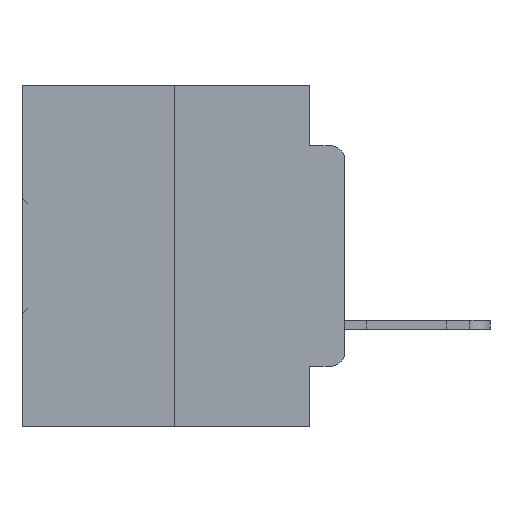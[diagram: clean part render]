
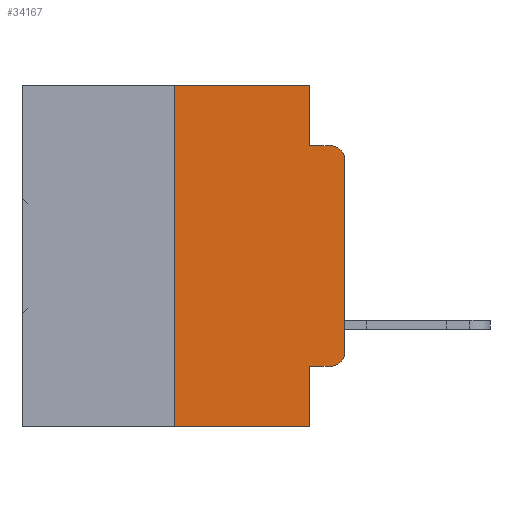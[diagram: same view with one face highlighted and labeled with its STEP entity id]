
A CAD part, left-side view. The second image highlights one B-rep face of the part: STEP entity #34167.
In plain terms, the highlighted planar face has unit normal (-1, 0, 0).
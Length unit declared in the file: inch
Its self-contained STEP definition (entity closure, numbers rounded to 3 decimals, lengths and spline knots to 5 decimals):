
#815 = VERTEX_POINT ( 'NONE', #9999 ) ;
#1784 = AXIS2_PLACEMENT_3D ( 'NONE', #13565, #32236, #16232 ) ;
#1846 = LINE ( 'NONE', #5525, #16604 ) ;
#2454 = CARTESIAN_POINT ( 'NONE',  ( 0., 0.473, -0.5 ) ) ;
#2669 = CARTESIAN_POINT ( 'NONE',  ( 0., 0.051, 0. ) ) ;
#2680 = VERTEX_POINT ( 'NONE', #14502 ) ;
#3505 = ORIENTED_EDGE ( 'NONE', *, *, #15313, .F. ) ;
#3794 = DIRECTION ( 'NONE',  ( 0., -1., 0. ) ) ;
#3886 = EDGE_CURVE ( 'NONE', #815, #17534, #33756, .T. ) ;
#4119 = CIRCLE ( 'NONE', #1784, 0.02 ) ;
#4231 = ORIENTED_EDGE ( 'NONE', *, *, #27863, .F. ) ;
#4337 = CARTESIAN_POINT ( 'NONE',  ( 0., 0.25, 0. ) ) ;
#5525 = CARTESIAN_POINT ( 'NONE',  ( 0., 0., 0. ) ) ;
#6463 = CARTESIAN_POINT ( 'NONE',  ( 0., 0.051, 0. ) ) ;
#6866 = VERTEX_POINT ( 'NONE', #31218 ) ;
#7298 = FACE_OUTER_BOUND ( 'NONE', #7932, .T. ) ;
#7543 = CARTESIAN_POINT ( 'NONE',  ( 0., 0., -0.1085 ) ) ;
#7589 = CARTESIAN_POINT ( 'NONE',  ( 0., 0., -0.3915 ) ) ;
#7918 = EDGE_CURVE ( 'NONE', #25588, #6866, #33479, .T. ) ;
#7932 = EDGE_LOOP ( 'NONE', ( #9572, #29184, #14953, #4231, #29340, #10903, #31826, #3505, #14131, #22045 ) ) ;
#8846 = CARTESIAN_POINT ( 'NONE',  ( 0., 0.051, -0.0885 ) ) ;
#9166 = DIRECTION ( 'NONE',  ( -1., 0., 0. ) ) ;
#9572 = ORIENTED_EDGE ( 'NONE', *, *, #12365, .T. ) ;
#9704 = AXIS2_PLACEMENT_3D ( 'NONE', #34174, #26301, #10127 ) ;
#9999 = CARTESIAN_POINT ( 'NONE',  ( 0., 0.051, -0.0885 ) ) ;
#10127 = DIRECTION ( 'NONE',  ( 0., 0., -1. ) ) ;
#10320 = DIRECTION ( 'NONE',  ( 0., -1., 0. ) ) ;
#10903 = ORIENTED_EDGE ( 'NONE', *, *, #7918, .F. ) ;
#10965 = EDGE_CURVE ( 'NONE', #11527, #17534, #4119, .T. ) ;
#11016 = VERTEX_POINT ( 'NONE', #32355 ) ;
#11527 = VERTEX_POINT ( 'NONE', #7543 ) ;
#12365 = EDGE_CURVE ( 'NONE', #23808, #11527, #1846, .T. ) ;
#12537 = LINE ( 'NONE', #17525, #17151 ) ;
#12842 = CARTESIAN_POINT ( 'NONE',  ( 0., 0.051, 0. ) ) ;
#13093 = EDGE_CURVE ( 'NONE', #25588, #21422, #21567, .T. ) ;
#13341 = VECTOR ( 'NONE', #33465, 39.37008 ) ;
#13565 = CARTESIAN_POINT ( 'NONE',  ( 0., 0.02, -0.1085 ) ) ;
#14131 = ORIENTED_EDGE ( 'NONE', *, *, #34041, .T. ) ;
#14473 = VECTOR ( 'NONE', #21647, 39.37008 ) ;
#14502 = CARTESIAN_POINT ( 'NONE',  ( 0., 0.051, -0.4115 ) ) ;
#14953 = ORIENTED_EDGE ( 'NONE', *, *, #3886, .F. ) ;
#15313 = EDGE_CURVE ( 'NONE', #2680, #21422, #33087, .T. ) ;
#15540 = DIRECTION ( 'NONE',  ( 0., 0., -1. ) ) ;
#16038 = CARTESIAN_POINT ( 'NONE',  ( 0., 0.051, -0.5 ) ) ;
#16232 = DIRECTION ( 'NONE',  ( 0., 0., -1. ) ) ;
#16604 = VECTOR ( 'NONE', #24638, 39.37008 ) ;
#16942 = VECTOR ( 'NONE', #23883, 39.37008 ) ;
#17151 = VECTOR ( 'NONE', #3794, 39.37008 ) ;
#17525 = CARTESIAN_POINT ( 'NONE',  ( 0., 0.051, -0.4115 ) ) ;
#17534 = VERTEX_POINT ( 'NONE', #20799 ) ;
#18224 = PLANE ( 'NONE',  #9704 ) ;
#18900 = VECTOR ( 'NONE', #15540, 39.37008 ) ;
#19289 = VECTOR ( 'NONE', #23483, 39.37008 ) ;
#19571 = VECTOR ( 'NONE', #10320, 39.37008 ) ;
#20799 = CARTESIAN_POINT ( 'NONE',  ( 0., 0.02, -0.0885 ) ) ;
#21422 = VERTEX_POINT ( 'NONE', #16038 ) ;
#21567 = LINE ( 'NONE', #2454, #14473 ) ;
#21647 = DIRECTION ( 'NONE',  ( 0., -1., 0. ) ) ;
#22045 = ORIENTED_EDGE ( 'NONE', *, *, #27207, .T. ) ;
#23483 = DIRECTION ( 'NONE',  ( 0., 0., 1. ) ) ;
#23808 = VERTEX_POINT ( 'NONE', #7589 ) ;
#23883 = DIRECTION ( 'NONE',  ( 0., -1., 0. ) ) ;
#23956 = VERTEX_POINT ( 'NONE', #2669 ) ;
#24638 = DIRECTION ( 'NONE',  ( 0., 0., 1. ) ) ;
#24974 = LINE ( 'NONE', #34374, #16942 ) ;
#25389 = CARTESIAN_POINT ( 'NONE',  ( 0., 0.02, -0.3915 ) ) ;
#25588 = VERTEX_POINT ( 'NONE', #34694 ) ;
#26301 = DIRECTION ( 'NONE',  ( 1., 0., 0. ) ) ;
#27207 = EDGE_CURVE ( 'NONE', #11016, #23808, #31590, .T. ) ;
#27453 = EDGE_CURVE ( 'NONE', #6866, #23956, #24974, .T. ) ;
#27839 = AXIS2_PLACEMENT_3D ( 'NONE', #25389, #9166, #28053 ) ;
#27863 = EDGE_CURVE ( 'NONE', #23956, #815, #34590, .T. ) ;
#28053 = DIRECTION ( 'NONE',  ( 0., 0., -1. ) ) ;
#29184 = ORIENTED_EDGE ( 'NONE', *, *, #10965, .T. ) ;
#29340 = ORIENTED_EDGE ( 'NONE', *, *, #27453, .F. ) ;
#31218 = CARTESIAN_POINT ( 'NONE',  ( 0., 0.25, 0. ) ) ;
#31590 = CIRCLE ( 'NONE', #27839, 0.02 ) ;
#31826 = ORIENTED_EDGE ( 'NONE', *, *, #13093, .T. ) ;
#32236 = DIRECTION ( 'NONE',  ( -1., 0., 0. ) ) ;
#32355 = CARTESIAN_POINT ( 'NONE',  ( 0., 0.02, -0.4115 ) ) ;
#33087 = LINE ( 'NONE', #12842, #18900 ) ;
#33465 = DIRECTION ( 'NONE',  ( 0., 0., -1. ) ) ;
#33479 = LINE ( 'NONE', #4337, #19289 ) ;
#33756 = LINE ( 'NONE', #8846, #19571 ) ;
#34041 = EDGE_CURVE ( 'NONE', #2680, #11016, #12537, .T. ) ;
#34167 = ADVANCED_FACE ( 'NONE', ( #7298 ), #18224, .F. ) ;
#34174 = CARTESIAN_POINT ( 'NONE',  ( 0., 0.473, 0. ) ) ;
#34374 = CARTESIAN_POINT ( 'NONE',  ( 0., 0.473, 0. ) ) ;
#34590 = LINE ( 'NONE', #6463, #13341 ) ;
#34694 = CARTESIAN_POINT ( 'NONE',  ( 0., 0.25, -0.5 ) ) ;
